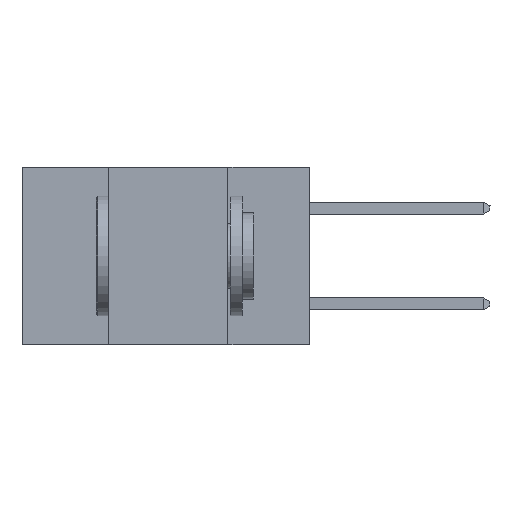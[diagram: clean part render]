
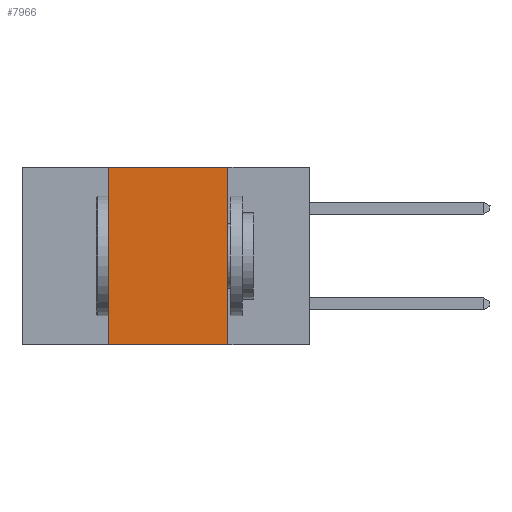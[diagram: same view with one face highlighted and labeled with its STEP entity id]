
A CAD part, left-side view. The second image highlights one B-rep face of the part: STEP entity #7966.
In plain terms, the highlighted planar face has unit normal (-1, 0, 0).
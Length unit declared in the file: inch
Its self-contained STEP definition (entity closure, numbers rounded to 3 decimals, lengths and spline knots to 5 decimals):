
#544 = DIRECTION ( 'NONE',  ( 0., 0., 1. ) ) ;
#1229 = CARTESIAN_POINT ( 'NONE',  ( 0., 0.6, -0.37 ) ) ;
#1724 = VECTOR ( 'NONE', #9869, 39.37008 ) ;
#1908 = LINE ( 'NONE', #6534, #1724 ) ;
#3342 = ORIENTED_EDGE ( 'NONE', *, *, #7914, .F. ) ;
#3418 = VECTOR ( 'NONE', #8266, 39.37008 ) ;
#3937 = LINE ( 'NONE', #1229, #3418 ) ;
#4049 = AXIS2_PLACEMENT_3D ( 'NONE', #12358, #8920, #12507 ) ;
#4305 = PLANE ( 'NONE',  #4049 ) ;
#4736 = VERTEX_POINT ( 'NONE', #12681 ) ;
#4739 = VECTOR ( 'NONE', #544, 39.37008 ) ;
#4769 = FACE_OUTER_BOUND ( 'NONE', #11783, .T. ) ;
#5494 = CARTESIAN_POINT ( 'NONE',  ( 0., 0.17, 0. ) ) ;
#6534 = CARTESIAN_POINT ( 'NONE',  ( 0., 0.6, 0. ) ) ;
#6651 = CARTESIAN_POINT ( 'NONE',  ( 0., 0.17, 0. ) ) ;
#7159 = VERTEX_POINT ( 'NONE', #5494 ) ;
#7423 = CARTESIAN_POINT ( 'NONE',  ( 0., 0.42, 0. ) ) ;
#7678 = ORIENTED_EDGE ( 'NONE', *, *, #13703, .F. ) ;
#7914 = EDGE_CURVE ( 'NONE', #10625, #7159, #1908, .T. ) ;
#7966 = ADVANCED_FACE ( 'NONE', ( #4769 ), #4305, .F. ) ;
#8266 = DIRECTION ( 'NONE',  ( 0., -1., 0. ) ) ;
#8645 = ORIENTED_EDGE ( 'NONE', *, *, #14249, .F. ) ;
#8920 = DIRECTION ( 'NONE',  ( 1., 0., 0. ) ) ;
#9143 = ORIENTED_EDGE ( 'NONE', *, *, #9300, .T. ) ;
#9300 = EDGE_CURVE ( 'NONE', #4736, #14493, #3937, .T. ) ;
#9869 = DIRECTION ( 'NONE',  ( 0., -1., 0. ) ) ;
#10495 = LINE ( 'NONE', #7423, #4739 ) ;
#10625 = VERTEX_POINT ( 'NONE', #14687 ) ;
#11677 = CARTESIAN_POINT ( 'NONE',  ( 0., 0.17, -0.37 ) ) ;
#11783 = EDGE_LOOP ( 'NONE', ( #8645, #3342, #7678, #9143 ) ) ;
#12358 = CARTESIAN_POINT ( 'NONE',  ( 0., 0.6, 0. ) ) ;
#12507 = DIRECTION ( 'NONE',  ( 0., 0., -1. ) ) ;
#12681 = CARTESIAN_POINT ( 'NONE',  ( 0., 0.42, -0.37 ) ) ;
#13703 = EDGE_CURVE ( 'NONE', #4736, #10625, #10495, .T. ) ;
#13726 = LINE ( 'NONE', #6651, #14260 ) ;
#14249 = EDGE_CURVE ( 'NONE', #7159, #14493, #13726, .T. ) ;
#14260 = VECTOR ( 'NONE', #14795, 39.37008 ) ;
#14493 = VERTEX_POINT ( 'NONE', #11677 ) ;
#14687 = CARTESIAN_POINT ( 'NONE',  ( 0., 0.42, 0. ) ) ;
#14795 = DIRECTION ( 'NONE',  ( 0., 0., -1. ) ) ;
